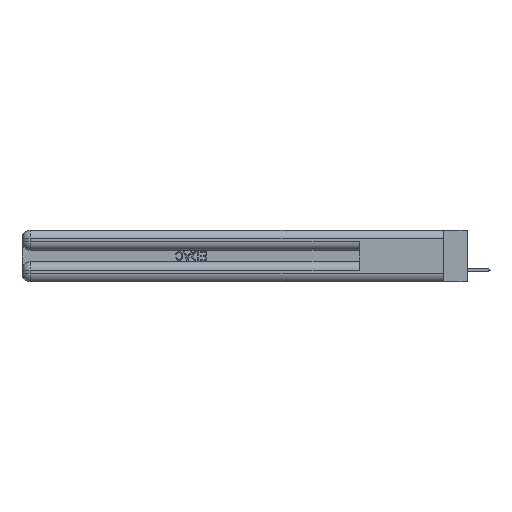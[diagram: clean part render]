
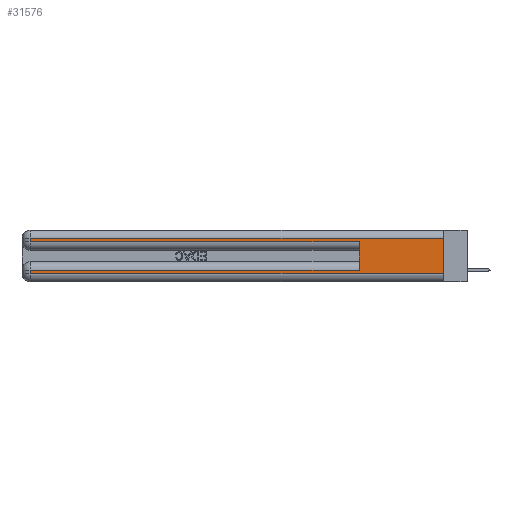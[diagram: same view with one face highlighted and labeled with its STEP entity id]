
A CAD part, left-side view. The second image highlights one B-rep face of the part: STEP entity #31576.
In plain terms, the highlighted planar face has unit normal (-1, 0, 0).
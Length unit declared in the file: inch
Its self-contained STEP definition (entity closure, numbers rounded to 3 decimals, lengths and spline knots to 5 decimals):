
#105 = ORIENTED_EDGE ( 'NONE', *, *, #15829, .T. ) ;
#575 = VERTEX_POINT ( 'NONE', #20793 ) ;
#1107 = ORIENTED_EDGE ( 'NONE', *, *, #3308, .T. ) ;
#2291 = VECTOR ( 'NONE', #21475, 39.37008 ) ;
#2901 = VERTEX_POINT ( 'NONE', #26612 ) ;
#3100 = CARTESIAN_POINT ( 'NONE',  ( 0., 0., 0.31 ) ) ;
#3308 = EDGE_CURVE ( 'NONE', #575, #2901, #32772, .T. ) ;
#5418 = DIRECTION ( 'NONE',  ( 0., 0., 1. ) ) ;
#6575 = DIRECTION ( 'NONE',  ( 1., 0., 0. ) ) ;
#7178 = CARTESIAN_POINT ( 'NONE',  ( 0., 2.94, 0.285 ) ) ;
#7591 = LINE ( 'NONE', #25924, #13597 ) ;
#9934 = VECTOR ( 'NONE', #23986, 39.37008 ) ;
#10406 = DIRECTION ( 'NONE',  ( 0., 0., -1. ) ) ;
#10414 = ORIENTED_EDGE ( 'NONE', *, *, #18406, .T. ) ;
#11238 = DIRECTION ( 'NONE',  ( 0., 0., -1. ) ) ;
#11787 = CARTESIAN_POINT ( 'NONE',  ( 0., 0., 0.085 ) ) ;
#11845 = ORIENTED_EDGE ( 'NONE', *, *, #24003, .F. ) ;
#13597 = VECTOR ( 'NONE', #5418, 39.37008 ) ;
#14188 = CARTESIAN_POINT ( 'NONE',  ( 0., 2.94, 0.37 ) ) ;
#14327 = CARTESIAN_POINT ( 'NONE',  ( 0., 0., 0.285 ) ) ;
#15829 = EDGE_CURVE ( 'NONE', #23482, #40599, #20816, .T. ) ;
#18146 = LINE ( 'NONE', #14188, #29964 ) ;
#18188 = VERTEX_POINT ( 'NONE', #33547 ) ;
#18406 = EDGE_CURVE ( 'NONE', #36360, #18188, #44694, .T. ) ;
#18417 = ORIENTED_EDGE ( 'NONE', *, *, #21048, .T. ) ;
#18551 = CARTESIAN_POINT ( 'NONE',  ( 0., 0., 0.31 ) ) ;
#19021 = VECTOR ( 'NONE', #39190, 39.37008 ) ;
#20392 = EDGE_CURVE ( 'NONE', #40599, #575, #18146, .T. ) ;
#20793 = CARTESIAN_POINT ( 'NONE',  ( 0., 2.94, 0.06 ) ) ;
#20816 = LINE ( 'NONE', #11787, #9934 ) ;
#21048 = EDGE_CURVE ( 'NONE', #26754, #36360, #41823, .T. ) ;
#21190 = EDGE_CURVE ( 'NONE', #32966, #26754, #44488, .T. ) ;
#21475 = DIRECTION ( 'NONE',  ( 0., -1., 0. ) ) ;
#21737 = VECTOR ( 'NONE', #11238, 39.37008 ) ;
#23287 = CARTESIAN_POINT ( 'NONE',  ( 0., 2.94, 0.31 ) ) ;
#23482 = VERTEX_POINT ( 'NONE', #23708 ) ;
#23708 = CARTESIAN_POINT ( 'NONE',  ( 0., 0.6, 0.085 ) ) ;
#23800 = EDGE_CURVE ( 'NONE', #32966, #2901, #27192, .T. ) ;
#23986 = DIRECTION ( 'NONE',  ( 0., 1., 0. ) ) ;
#24003 = EDGE_CURVE ( 'NONE', #23482, #18188, #7591, .T. ) ;
#24443 = AXIS2_PLACEMENT_3D ( 'NONE', #34847, #6575, #10406 ) ;
#25324 = FACE_OUTER_BOUND ( 'NONE', #36243, .T. ) ;
#25924 = CARTESIAN_POINT ( 'NONE',  ( 0., 0.6, 0.145 ) ) ;
#26612 = CARTESIAN_POINT ( 'NONE',  ( 0., 0., 0.06 ) ) ;
#26754 = VERTEX_POINT ( 'NONE', #23287 ) ;
#27192 = LINE ( 'NONE', #39630, #21737 ) ;
#27387 = PLANE ( 'NONE',  #24443 ) ;
#28269 = CARTESIAN_POINT ( 'NONE',  ( 0., 2.94, 0.37 ) ) ;
#28419 = DIRECTION ( 'NONE',  ( 0., 0., -1. ) ) ;
#29964 = VECTOR ( 'NONE', #31656, 39.37008 ) ;
#30507 = DIRECTION ( 'NONE',  ( 0., -1., 0. ) ) ;
#31576 = ADVANCED_FACE ( 'NONE', ( #25324 ), #27387, .F. ) ;
#31656 = DIRECTION ( 'NONE',  ( 0., 0., -1. ) ) ;
#32772 = LINE ( 'NONE', #37569, #33342 ) ;
#32966 = VERTEX_POINT ( 'NONE', #3100 ) ;
#33342 = VECTOR ( 'NONE', #30507, 39.37008 ) ;
#33547 = CARTESIAN_POINT ( 'NONE',  ( 0., 0.6, 0.285 ) ) ;
#33703 = ORIENTED_EDGE ( 'NONE', *, *, #23800, .F. ) ;
#34847 = CARTESIAN_POINT ( 'NONE',  ( 0., 0., 0.37 ) ) ;
#35327 = ORIENTED_EDGE ( 'NONE', *, *, #21190, .T. ) ;
#36243 = EDGE_LOOP ( 'NONE', ( #33703, #35327, #18417, #10414, #11845, #105, #37670, #1107 ) ) ;
#36360 = VERTEX_POINT ( 'NONE', #7178 ) ;
#37569 = CARTESIAN_POINT ( 'NONE',  ( 0., 0., 0.06 ) ) ;
#37670 = ORIENTED_EDGE ( 'NONE', *, *, #20392, .T. ) ;
#39190 = DIRECTION ( 'NONE',  ( 0., 1., 0. ) ) ;
#39630 = CARTESIAN_POINT ( 'NONE',  ( 0., 0., 0.37 ) ) ;
#40186 = VECTOR ( 'NONE', #28419, 39.37008 ) ;
#40599 = VERTEX_POINT ( 'NONE', #43934 ) ;
#41823 = LINE ( 'NONE', #28269, #40186 ) ;
#43934 = CARTESIAN_POINT ( 'NONE',  ( 0., 2.94, 0.085 ) ) ;
#44488 = LINE ( 'NONE', #18551, #19021 ) ;
#44694 = LINE ( 'NONE', #14327, #2291 ) ;
